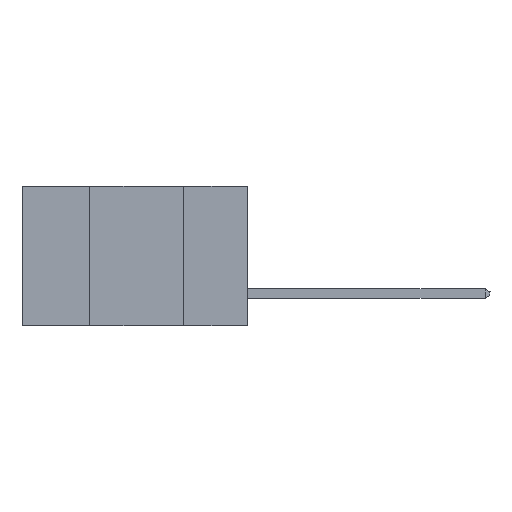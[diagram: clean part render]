
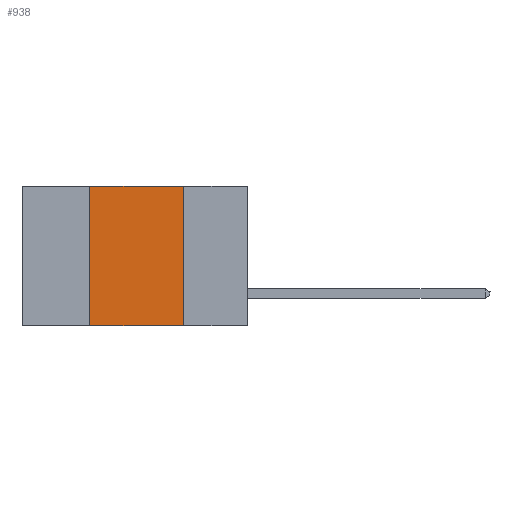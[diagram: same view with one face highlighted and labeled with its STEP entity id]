
A CAD part, left-side view. The second image highlights one B-rep face of the part: STEP entity #938.
In plain terms, the highlighted planar face has unit normal (-1, 0, 0).
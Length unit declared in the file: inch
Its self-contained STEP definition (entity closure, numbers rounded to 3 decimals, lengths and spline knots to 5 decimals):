
#835 = CARTESIAN_POINT ( 'NONE',  ( 0., 0.6, 0. ) ) ;
#929 = VERTEX_POINT ( 'NONE', #6620 ) ;
#938 = ADVANCED_FACE ( 'NONE', ( #6713 ), #16628, .F. ) ;
#1106 = DIRECTION ( 'NONE',  ( 0., -1., 0. ) ) ;
#1392 = ORIENTED_EDGE ( 'NONE', *, *, #3000, .F. ) ;
#2222 = DIRECTION ( 'NONE',  ( 1., 0., 0. ) ) ;
#2360 = DIRECTION ( 'NONE',  ( 0., 0., 1. ) ) ;
#2703 = CARTESIAN_POINT ( 'NONE',  ( 0., 0.42, -0.37 ) ) ;
#2735 = VERTEX_POINT ( 'NONE', #4342 ) ;
#3000 = EDGE_CURVE ( 'NONE', #12606, #929, #5177, .T. ) ;
#3187 = AXIS2_PLACEMENT_3D ( 'NONE', #13911, #2222, #16448 ) ;
#3190 = DIRECTION ( 'NONE',  ( 0., 0., -1. ) ) ;
#3593 = DIRECTION ( 'NONE',  ( 0., -1., 0. ) ) ;
#4117 = VERTEX_POINT ( 'NONE', #13082 ) ;
#4342 = CARTESIAN_POINT ( 'NONE',  ( 0., 0.17, 0. ) ) ;
#4901 = CARTESIAN_POINT ( 'NONE',  ( 0., 0.6, -0.37 ) ) ;
#5177 = LINE ( 'NONE', #13688, #14733 ) ;
#5541 = ORIENTED_EDGE ( 'NONE', *, *, #11512, .F. ) ;
#5699 = ORIENTED_EDGE ( 'NONE', *, *, #16754, .F. ) ;
#5790 = VECTOR ( 'NONE', #1106, 39.37008 ) ;
#6620 = CARTESIAN_POINT ( 'NONE',  ( 0., 0.42, 0. ) ) ;
#6713 = FACE_OUTER_BOUND ( 'NONE', #16966, .T. ) ;
#10381 = VECTOR ( 'NONE', #3190, 39.37008 ) ;
#10828 = LINE ( 'NONE', #835, #5790 ) ;
#11512 = EDGE_CURVE ( 'NONE', #2735, #4117, #16101, .T. ) ;
#11678 = CARTESIAN_POINT ( 'NONE',  ( 0., 0.17, -0.37 ) ) ;
#12606 = VERTEX_POINT ( 'NONE', #2703 ) ;
#13082 = CARTESIAN_POINT ( 'NONE',  ( 0., 0.17, -0.37 ) ) ;
#13688 = CARTESIAN_POINT ( 'NONE',  ( 0., 0.42, -0.37 ) ) ;
#13911 = CARTESIAN_POINT ( 'NONE',  ( 0., 0.6, 0. ) ) ;
#14733 = VECTOR ( 'NONE', #2360, 39.37008 ) ;
#14960 = VECTOR ( 'NONE', #3593, 39.37008 ) ;
#15833 = ORIENTED_EDGE ( 'NONE', *, *, #16119, .T. ) ;
#16101 = LINE ( 'NONE', #11678, #10381 ) ;
#16119 = EDGE_CURVE ( 'NONE', #12606, #4117, #16303, .T. ) ;
#16303 = LINE ( 'NONE', #4901, #14960 ) ;
#16448 = DIRECTION ( 'NONE',  ( 0., 0., -1. ) ) ;
#16628 = PLANE ( 'NONE',  #3187 ) ;
#16754 = EDGE_CURVE ( 'NONE', #929, #2735, #10828, .T. ) ;
#16966 = EDGE_LOOP ( 'NONE', ( #5541, #5699, #1392, #15833 ) ) ;
